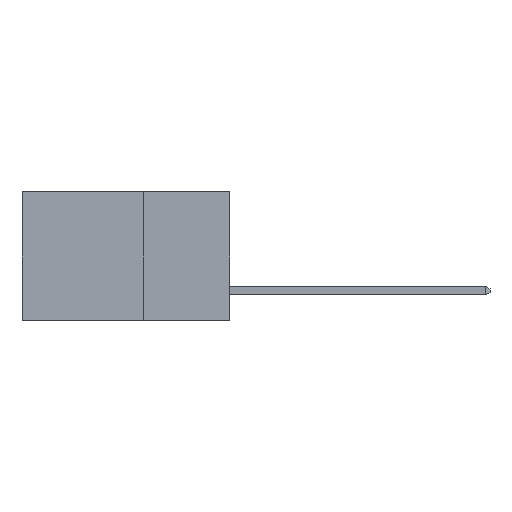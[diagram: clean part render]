
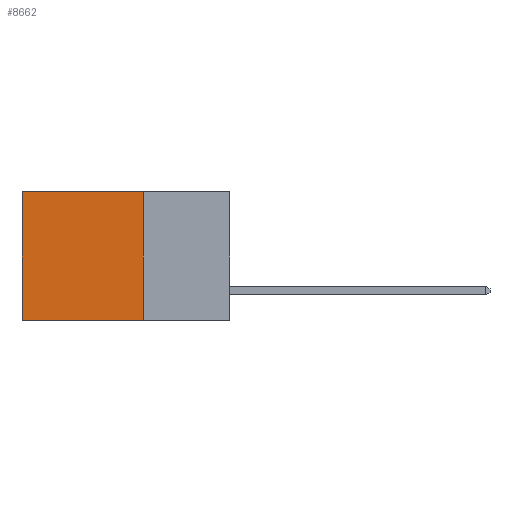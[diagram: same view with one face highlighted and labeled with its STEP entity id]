
A CAD part, left-side view. The second image highlights one B-rep face of the part: STEP entity #8662.
In plain terms, the highlighted planar face has unit normal (-1, 0, 0).
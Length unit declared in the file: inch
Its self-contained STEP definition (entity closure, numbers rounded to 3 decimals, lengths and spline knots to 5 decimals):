
#217 = VERTEX_POINT ( 'NONE', #3247 ) ;
#347 = EDGE_CURVE ( 'NONE', #611, #1354, #6173, .T. ) ;
#543 = CARTESIAN_POINT ( 'NONE',  ( 0.2615, 0.25, 0. ) ) ;
#611 = VERTEX_POINT ( 'NONE', #10849 ) ;
#791 = CARTESIAN_POINT ( 'NONE',  ( 0.2615, 0.25, -0.37 ) ) ;
#799 = CARTESIAN_POINT ( 'NONE',  ( 0.2615, 0.25, -0.37 ) ) ;
#809 = LINE ( 'NONE', #799, #3707 ) ;
#1155 = DIRECTION ( 'NONE',  ( 0., 1., 0. ) ) ;
#1354 = VERTEX_POINT ( 'NONE', #3616 ) ;
#1567 = DIRECTION ( 'NONE',  ( 0., 1., 0. ) ) ;
#1614 = EDGE_CURVE ( 'NONE', #4844, #611, #809, .T. ) ;
#2037 = AXIS2_PLACEMENT_3D ( 'NONE', #8281, #9126, #4098 ) ;
#2038 = DIRECTION ( 'NONE',  ( 0., 0., -1. ) ) ;
#2244 = PLANE ( 'NONE',  #2037 ) ;
#2569 = LINE ( 'NONE', #4355, #11177 ) ;
#3247 = CARTESIAN_POINT ( 'NONE',  ( 0.2615, 0.6, 0. ) ) ;
#3616 = CARTESIAN_POINT ( 'NONE',  ( 0.2615, 0.6, -0.37 ) ) ;
#3667 = CARTESIAN_POINT ( 'NONE',  ( 0.2615, 0.25, 0. ) ) ;
#3707 = VECTOR ( 'NONE', #2038, 39.37008 ) ;
#3875 = EDGE_CURVE ( 'NONE', #4844, #217, #11000, .T. ) ;
#4098 = DIRECTION ( 'NONE',  ( 0., 0., -1. ) ) ;
#4355 = CARTESIAN_POINT ( 'NONE',  ( 0.2615, 0.6, -0.37 ) ) ;
#4357 = DIRECTION ( 'NONE',  ( 0., 0., -1. ) ) ;
#4844 = VERTEX_POINT ( 'NONE', #543 ) ;
#5090 = ORIENTED_EDGE ( 'NONE', *, *, #7647, .T. ) ;
#5113 = ORIENTED_EDGE ( 'NONE', *, *, #347, .F. ) ;
#5119 = ORIENTED_EDGE ( 'NONE', *, *, #1614, .F. ) ;
#5122 = ORIENTED_EDGE ( 'NONE', *, *, #3875, .T. ) ;
#5695 = EDGE_LOOP ( 'NONE', ( #5090, #5113, #5119, #5122 ) ) ;
#6173 = LINE ( 'NONE', #791, #10281 ) ;
#6713 = VECTOR ( 'NONE', #1567, 39.37008 ) ;
#7159 = FACE_OUTER_BOUND ( 'NONE', #5695, .T. ) ;
#7647 = EDGE_CURVE ( 'NONE', #217, #1354, #2569, .T. ) ;
#8281 = CARTESIAN_POINT ( 'NONE',  ( 0.2615, 0.25, -0.37 ) ) ;
#8662 = ADVANCED_FACE ( 'NONE', ( #7159 ), #2244, .F. ) ;
#9126 = DIRECTION ( 'NONE',  ( 1., 0., 0. ) ) ;
#10281 = VECTOR ( 'NONE', #1155, 39.37008 ) ;
#10849 = CARTESIAN_POINT ( 'NONE',  ( 0.2615, 0.25, -0.37 ) ) ;
#11000 = LINE ( 'NONE', #3667, #6713 ) ;
#11177 = VECTOR ( 'NONE', #4357, 39.37008 ) ;
